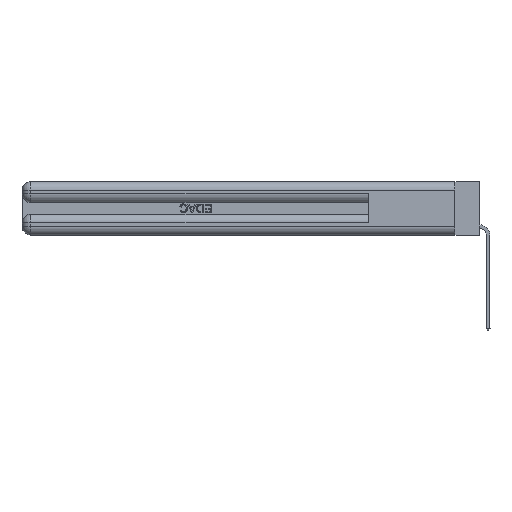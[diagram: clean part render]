
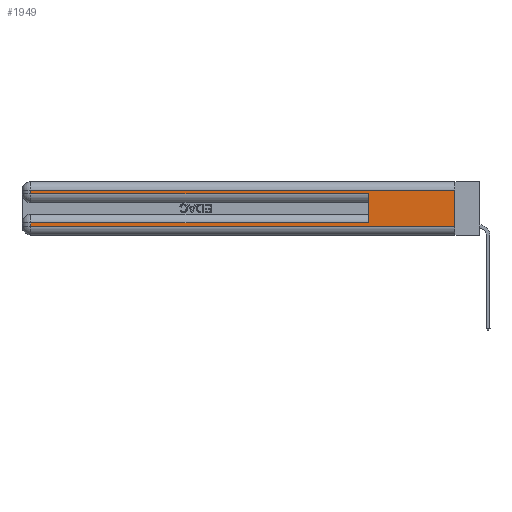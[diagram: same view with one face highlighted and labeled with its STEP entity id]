
A CAD part, left-side view. The second image highlights one B-rep face of the part: STEP entity #1949.
In plain terms, the highlighted planar face has unit normal (-1, 0, 0).
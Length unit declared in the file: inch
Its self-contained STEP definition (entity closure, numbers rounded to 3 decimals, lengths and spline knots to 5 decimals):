
#156 = CARTESIAN_POINT ( 'NONE',  ( 0., 0., 0.06 ) ) ;
#560 = VERTEX_POINT ( 'NONE', #10841 ) ;
#577 = VERTEX_POINT ( 'NONE', #15267 ) ;
#715 = CARTESIAN_POINT ( 'NONE',  ( 0., 2.94, 0.37 ) ) ;
#867 = CARTESIAN_POINT ( 'NONE',  ( 0., 0.6, 0.085 ) ) ;
#1339 = EDGE_CURVE ( 'NONE', #24908, #577, #19471, .T. ) ;
#1504 = ORIENTED_EDGE ( 'NONE', *, *, #1339, .T. ) ;
#1949 = ADVANCED_FACE ( 'NONE', ( #16104 ), #17626, .F. ) ;
#2207 = LINE ( 'NONE', #20891, #5168 ) ;
#2574 = CARTESIAN_POINT ( 'NONE',  ( 0., 0., 0.06 ) ) ;
#2688 = ORIENTED_EDGE ( 'NONE', *, *, #20521, .T. ) ;
#2765 = DIRECTION ( 'NONE',  ( 0., 0., -1. ) ) ;
#3167 = VERTEX_POINT ( 'NONE', #13289 ) ;
#3277 = CARTESIAN_POINT ( 'NONE',  ( 0., 2.94, 0.31 ) ) ;
#3307 = VECTOR ( 'NONE', #26518, 39.37008 ) ;
#3997 = CARTESIAN_POINT ( 'NONE',  ( 0., 0., 0.37 ) ) ;
#4176 = DIRECTION ( 'NONE',  ( 0., 0., -1. ) ) ;
#4612 = CARTESIAN_POINT ( 'NONE',  ( 0., 0., 0.085 ) ) ;
#4826 = LINE ( 'NONE', #2574, #6302 ) ;
#5168 = VECTOR ( 'NONE', #21430, 39.37008 ) ;
#5386 = CARTESIAN_POINT ( 'NONE',  ( 0., 0., 0.37 ) ) ;
#6302 = VECTOR ( 'NONE', #10820, 39.37008 ) ;
#6642 = CARTESIAN_POINT ( 'NONE',  ( 0., 0., 0.31 ) ) ;
#7224 = DIRECTION ( 'NONE',  ( 1., 0., 0. ) ) ;
#7662 = EDGE_CURVE ( 'NONE', #560, #3167, #2207, .T. ) ;
#8155 = VERTEX_POINT ( 'NONE', #16518 ) ;
#8654 = ORIENTED_EDGE ( 'NONE', *, *, #7662, .T. ) ;
#8766 = ORIENTED_EDGE ( 'NONE', *, *, #23681, .F. ) ;
#9604 = VERTEX_POINT ( 'NONE', #3277 ) ;
#10357 = VERTEX_POINT ( 'NONE', #867 ) ;
#10813 = LINE ( 'NONE', #6642, #12405 ) ;
#10820 = DIRECTION ( 'NONE',  ( 0., -1., 0. ) ) ;
#10841 = CARTESIAN_POINT ( 'NONE',  ( 0., 2.94, 0.285 ) ) ;
#10981 = VECTOR ( 'NONE', #4176, 39.37008 ) ;
#11008 = VECTOR ( 'NONE', #13116, 39.37008 ) ;
#11488 = VERTEX_POINT ( 'NONE', #156 ) ;
#12405 = VECTOR ( 'NONE', #23609, 39.37008 ) ;
#12518 = DIRECTION ( 'NONE',  ( 0., 0., -1. ) ) ;
#12652 = VECTOR ( 'NONE', #12518, 39.37008 ) ;
#13116 = DIRECTION ( 'NONE',  ( 0., 1., 0. ) ) ;
#13289 = CARTESIAN_POINT ( 'NONE',  ( 0., 0.6, 0.285 ) ) ;
#13552 = EDGE_CURVE ( 'NONE', #8155, #9604, #10813, .T. ) ;
#13621 = DIRECTION ( 'NONE',  ( 0., 0., -1. ) ) ;
#15169 = LINE ( 'NONE', #4612, #11008 ) ;
#15267 = CARTESIAN_POINT ( 'NONE',  ( 0., 2.94, 0.06 ) ) ;
#16104 = FACE_OUTER_BOUND ( 'NONE', #20859, .T. ) ;
#16518 = CARTESIAN_POINT ( 'NONE',  ( 0., 0., 0.31 ) ) ;
#16559 = LINE ( 'NONE', #25059, #10981 ) ;
#17476 = EDGE_CURVE ( 'NONE', #10357, #24908, #15169, .T. ) ;
#17626 = PLANE ( 'NONE',  #23579 ) ;
#18341 = CARTESIAN_POINT ( 'NONE',  ( 0., 2.94, 0.085 ) ) ;
#18501 = ORIENTED_EDGE ( 'NONE', *, *, #13552, .T. ) ;
#19471 = LINE ( 'NONE', #715, #19975 ) ;
#19931 = CARTESIAN_POINT ( 'NONE',  ( 0., 0.6, 0.145 ) ) ;
#19975 = VECTOR ( 'NONE', #2765, 39.37008 ) ;
#20220 = LINE ( 'NONE', #19931, #3307 ) ;
#20521 = EDGE_CURVE ( 'NONE', #577, #11488, #4826, .T. ) ;
#20859 = EDGE_LOOP ( 'NONE', ( #8766, #18501, #23274, #8654, #25759, #26529, #1504, #2688 ) ) ;
#20891 = CARTESIAN_POINT ( 'NONE',  ( 0., 0., 0.285 ) ) ;
#21201 = EDGE_CURVE ( 'NONE', #9604, #560, #16559, .T. ) ;
#21430 = DIRECTION ( 'NONE',  ( 0., -1., 0. ) ) ;
#23058 = LINE ( 'NONE', #3997, #12652 ) ;
#23274 = ORIENTED_EDGE ( 'NONE', *, *, #21201, .T. ) ;
#23579 = AXIS2_PLACEMENT_3D ( 'NONE', #5386, #7224, #13621 ) ;
#23609 = DIRECTION ( 'NONE',  ( 0., 1., 0. ) ) ;
#23681 = EDGE_CURVE ( 'NONE', #8155, #11488, #23058, .T. ) ;
#24236 = EDGE_CURVE ( 'NONE', #10357, #3167, #20220, .T. ) ;
#24908 = VERTEX_POINT ( 'NONE', #18341 ) ;
#25059 = CARTESIAN_POINT ( 'NONE',  ( 0., 2.94, 0.37 ) ) ;
#25759 = ORIENTED_EDGE ( 'NONE', *, *, #24236, .F. ) ;
#26518 = DIRECTION ( 'NONE',  ( 0., 0., 1. ) ) ;
#26529 = ORIENTED_EDGE ( 'NONE', *, *, #17476, .T. ) ;
